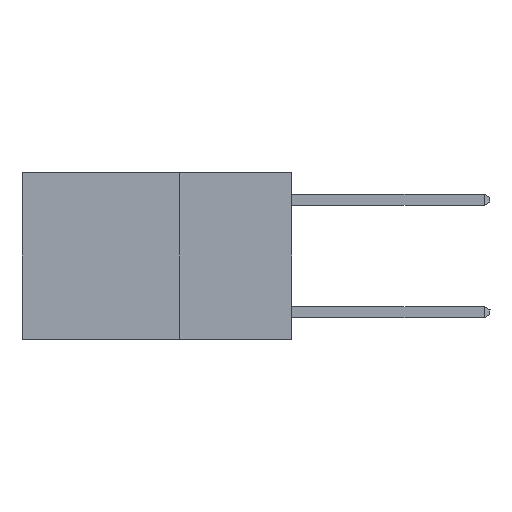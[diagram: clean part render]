
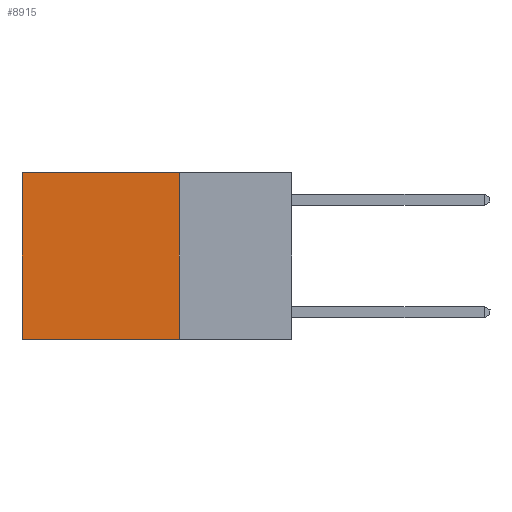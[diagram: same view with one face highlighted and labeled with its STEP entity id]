
A CAD part, left-side view. The second image highlights one B-rep face of the part: STEP entity #8915.
In plain terms, the highlighted planar face has unit normal (-1, 0, 0).
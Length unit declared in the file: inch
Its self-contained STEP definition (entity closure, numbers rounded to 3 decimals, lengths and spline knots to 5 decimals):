
#778 = LINE ( 'NONE', #3585, #8796 ) ;
#865 = DIRECTION ( 'NONE',  ( 0., 0., -1. ) ) ;
#1008 = VERTEX_POINT ( 'NONE', #12959 ) ;
#1057 = ORIENTED_EDGE ( 'NONE', *, *, #8962, .F. ) ;
#1101 = DIRECTION ( 'NONE',  ( 0., 1., 0. ) ) ;
#3199 = VERTEX_POINT ( 'NONE', #31618 ) ;
#3585 = CARTESIAN_POINT ( 'NONE',  ( 0.2625, 0.25, 0. ) ) ;
#3643 = DIRECTION ( 'NONE',  ( 0., 1., 0. ) ) ;
#4138 = DIRECTION ( 'NONE',  ( 1., 0., 0. ) ) ;
#5049 = ORIENTED_EDGE ( 'NONE', *, *, #27345, .F. ) ;
#5818 = EDGE_CURVE ( 'NONE', #1008, #3199, #23342, .T. ) ;
#6137 = LINE ( 'NONE', #21739, #25075 ) ;
#6293 = DIRECTION ( 'NONE',  ( 0., 0., -1. ) ) ;
#8796 = VECTOR ( 'NONE', #1101, 39.37008 ) ;
#8915 = ADVANCED_FACE ( 'NONE', ( #21417 ), #21915, .F. ) ;
#8962 = EDGE_CURVE ( 'NONE', #13169, #3199, #6137, .T. ) ;
#11293 = CARTESIAN_POINT ( 'NONE',  ( 0.2625, 0.25, 0. ) ) ;
#12761 = VECTOR ( 'NONE', #31147, 39.37008 ) ;
#12959 = CARTESIAN_POINT ( 'NONE',  ( 0.2625, 0.6, 0. ) ) ;
#13169 = VERTEX_POINT ( 'NONE', #27348 ) ;
#14977 = ORIENTED_EDGE ( 'NONE', *, *, #29580, .T. ) ;
#16135 = CARTESIAN_POINT ( 'NONE',  ( 0.2625, 0.25, 0. ) ) ;
#18036 = CARTESIAN_POINT ( 'NONE',  ( 0.2625, 0.6, 0. ) ) ;
#18705 = EDGE_LOOP ( 'NONE', ( #19634, #1057, #5049, #14977 ) ) ;
#19634 = ORIENTED_EDGE ( 'NONE', *, *, #5818, .T. ) ;
#20665 = VERTEX_POINT ( 'NONE', #26344 ) ;
#20836 = AXIS2_PLACEMENT_3D ( 'NONE', #11293, #4138, #6293 ) ;
#21417 = FACE_OUTER_BOUND ( 'NONE', #18705, .T. ) ;
#21739 = CARTESIAN_POINT ( 'NONE',  ( 0.2625, 0.25, -0.37 ) ) ;
#21915 = PLANE ( 'NONE',  #20836 ) ;
#23342 = LINE ( 'NONE', #18036, #12761 ) ;
#25075 = VECTOR ( 'NONE', #3643, 39.37008 ) ;
#26344 = CARTESIAN_POINT ( 'NONE',  ( 0.2625, 0.25, 0. ) ) ;
#27345 = EDGE_CURVE ( 'NONE', #20665, #13169, #31571, .T. ) ;
#27348 = CARTESIAN_POINT ( 'NONE',  ( 0.2625, 0.25, -0.37 ) ) ;
#29580 = EDGE_CURVE ( 'NONE', #20665, #1008, #778, .T. ) ;
#31147 = DIRECTION ( 'NONE',  ( 0., 0., -1. ) ) ;
#31571 = LINE ( 'NONE', #16135, #32107 ) ;
#31618 = CARTESIAN_POINT ( 'NONE',  ( 0.2625, 0.6, -0.37 ) ) ;
#32107 = VECTOR ( 'NONE', #865, 39.37008 ) ;
